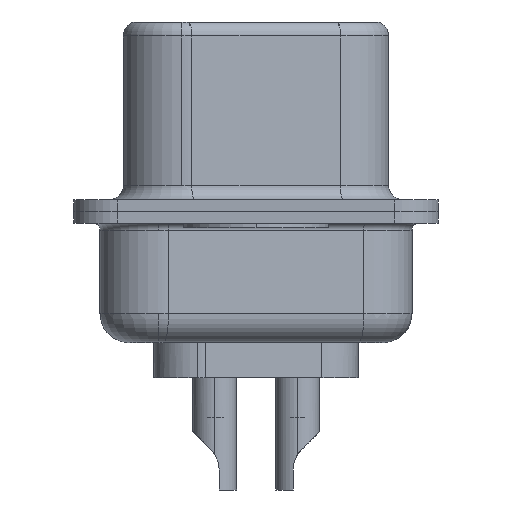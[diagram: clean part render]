
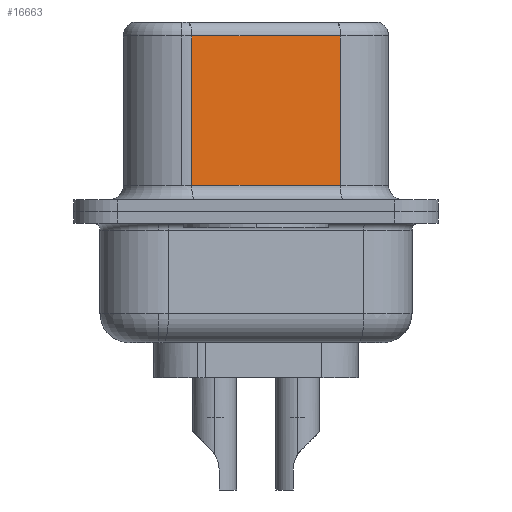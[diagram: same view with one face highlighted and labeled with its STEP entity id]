
A CAD part, left-side view. The second image highlights one B-rep face of the part: STEP entity #16663.
In plain terms, the highlighted planar face has unit normal (-0.985, -0.174, 0).
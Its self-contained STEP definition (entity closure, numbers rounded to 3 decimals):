
#590 = DIRECTION ( 'NONE',  ( 0., 0., -1. ) ) ;
#1134 = VECTOR ( 'NONE', #590, 1000. ) ;
#1248 = ORIENTED_EDGE ( 'NONE', *, *, #5174, .T. ) ;
#2155 = DIRECTION ( 'NONE',  ( -0.174, 0.985, 0. ) ) ;
#3212 = FACE_OUTER_BOUND ( 'NONE', #11265, .T. ) ;
#3436 = DIRECTION ( 'NONE',  ( 0.174, -0.985, 0. ) ) ;
#4750 = VERTEX_POINT ( 'NONE', #19507 ) ;
#5174 = EDGE_CURVE ( 'NONE', #6475, #4750, #11940, .T. ) ;
#5713 = VECTOR ( 'NONE', #2155, 1000. ) ;
#6475 = VERTEX_POINT ( 'NONE', #8315 ) ;
#8051 = VECTOR ( 'NONE', #21606, 1000. ) ;
#8315 = CARTESIAN_POINT ( 'NONE',  ( 3.68, 2.203, 0.9 ) ) ;
#8994 = DIRECTION ( 'NONE',  ( -0.174, 0.985, 0. ) ) ;
#9108 = EDGE_CURVE ( 'NONE', #14083, #6475, #23277, .T. ) ;
#10005 = ORIENTED_EDGE ( 'NONE', *, *, #16899, .F. ) ;
#10222 = ORIENTED_EDGE ( 'NONE', *, *, #19768, .T. ) ;
#10756 = CARTESIAN_POINT ( 'NONE',  ( 4.58, -2.897, 6.52 ) ) ;
#10994 = CARTESIAN_POINT ( 'NONE',  ( 3.68, 2.203, 6.52 ) ) ;
#11265 = EDGE_LOOP ( 'NONE', ( #10005, #10222, #14064, #1248 ) ) ;
#11545 = VERTEX_POINT ( 'NONE', #18673 ) ;
#11940 = LINE ( 'NONE', #19478, #19985 ) ;
#12072 = AXIS2_PLACEMENT_3D ( 'NONE', #10756, #12178, #8994 ) ;
#12178 = DIRECTION ( 'NONE',  ( 0.985, 0.174, 0. ) ) ;
#14064 = ORIENTED_EDGE ( 'NONE', *, *, #9108, .T. ) ;
#14083 = VERTEX_POINT ( 'NONE', #14477 ) ;
#14477 = CARTESIAN_POINT ( 'NONE',  ( 3.68, 2.203, 6.02 ) ) ;
#16081 = LINE ( 'NONE', #19721, #5713 ) ;
#16663 = ADVANCED_FACE ( 'NONE', ( #3212 ), #17722, .F. ) ;
#16899 = EDGE_CURVE ( 'NONE', #11545, #4750, #21726, .T. ) ;
#17722 = PLANE ( 'NONE',  #12072 ) ;
#18186 = CARTESIAN_POINT ( 'NONE',  ( 4.58, -2.897, 6.52 ) ) ;
#18673 = CARTESIAN_POINT ( 'NONE',  ( 4.58, -2.897, 6.02 ) ) ;
#19478 = CARTESIAN_POINT ( 'NONE',  ( 4.58, -2.897, 0.9 ) ) ;
#19507 = CARTESIAN_POINT ( 'NONE',  ( 4.58, -2.897, 0.9 ) ) ;
#19721 = CARTESIAN_POINT ( 'NONE',  ( 4.58, -2.897, 6.02 ) ) ;
#19768 = EDGE_CURVE ( 'NONE', #11545, #14083, #16081, .T. ) ;
#19985 = VECTOR ( 'NONE', #3436, 1000. ) ;
#21606 = DIRECTION ( 'NONE',  ( 0., 0., -1. ) ) ;
#21726 = LINE ( 'NONE', #18186, #1134 ) ;
#23277 = LINE ( 'NONE', #10994, #8051 ) ;
